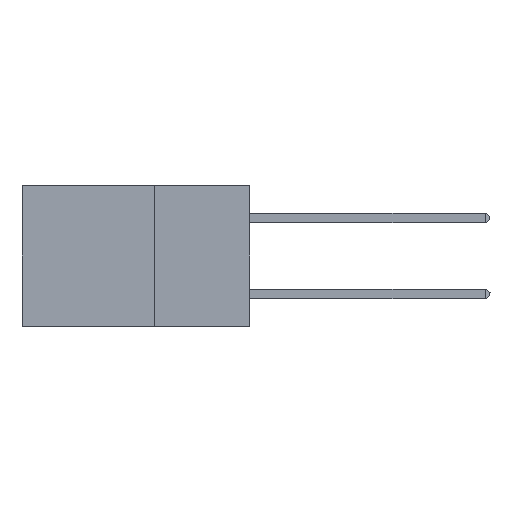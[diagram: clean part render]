
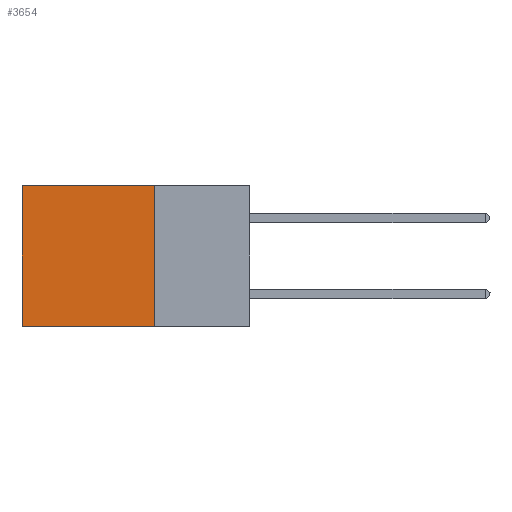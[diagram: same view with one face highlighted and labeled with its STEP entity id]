
A CAD part, left-side view. The second image highlights one B-rep face of the part: STEP entity #3654.
In plain terms, the highlighted planar face has unit normal (-1, 0, 0).
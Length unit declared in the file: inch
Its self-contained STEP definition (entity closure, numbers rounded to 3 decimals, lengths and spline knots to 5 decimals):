
#34 = LINE ( 'NONE', #11631, #18274 ) ;
#37 = PLANE ( 'NONE',  #7152 ) ;
#3406 = CARTESIAN_POINT ( 'NONE',  ( 0.2875, 0.25, 0. ) ) ;
#3477 = DIRECTION ( 'NONE',  ( 1., 0., 0. ) ) ;
#3566 = CARTESIAN_POINT ( 'NONE',  ( 0.2875, 0.25, 0. ) ) ;
#3654 = ADVANCED_FACE ( 'NONE', ( #11152 ), #37, .F. ) ;
#4020 = CARTESIAN_POINT ( 'NONE',  ( 0.2875, 0.6, 0. ) ) ;
#5907 = DIRECTION ( 'NONE',  ( 0., 1., 0. ) ) ;
#6200 = VERTEX_POINT ( 'NONE', #18949 ) ;
#6366 = VERTEX_POINT ( 'NONE', #14216 ) ;
#6969 = EDGE_CURVE ( 'NONE', #6200, #6366, #34, .T. ) ;
#7152 = AXIS2_PLACEMENT_3D ( 'NONE', #3566, #3477, #12568 ) ;
#7919 = ORIENTED_EDGE ( 'NONE', *, *, #6969, .T. ) ;
#9096 = EDGE_CURVE ( 'NONE', #6200, #17278, #19017, .T. ) ;
#9448 = ORIENTED_EDGE ( 'NONE', *, *, #17090, .T. ) ;
#9589 = DIRECTION ( 'NONE',  ( 0., 0., -1. ) ) ;
#9813 = LINE ( 'NONE', #22398, #17381 ) ;
#11152 = FACE_OUTER_BOUND ( 'NONE', #14545, .T. ) ;
#11631 = CARTESIAN_POINT ( 'NONE',  ( 0.2875, 0.25, 0. ) ) ;
#12011 = EDGE_CURVE ( 'NONE', #17278, #15014, #9813, .T. ) ;
#12568 = DIRECTION ( 'NONE',  ( 0., 0., -1. ) ) ;
#13454 = DIRECTION ( 'NONE',  ( 0., 1., 0. ) ) ;
#13642 = VECTOR ( 'NONE', #9589, 39.37008 ) ;
#14216 = CARTESIAN_POINT ( 'NONE',  ( 0.2875, 0.6, 0. ) ) ;
#14481 = LINE ( 'NONE', #4020, #13642 ) ;
#14545 = EDGE_LOOP ( 'NONE', ( #9448, #15467, #14942, #7919 ) ) ;
#14942 = ORIENTED_EDGE ( 'NONE', *, *, #9096, .F. ) ;
#15014 = VERTEX_POINT ( 'NONE', #22683 ) ;
#15467 = ORIENTED_EDGE ( 'NONE', *, *, #12011, .F. ) ;
#16002 = CARTESIAN_POINT ( 'NONE',  ( 0.2875, 0.25, -0.37 ) ) ;
#17090 = EDGE_CURVE ( 'NONE', #6366, #15014, #14481, .T. ) ;
#17278 = VERTEX_POINT ( 'NONE', #16002 ) ;
#17381 = VECTOR ( 'NONE', #5907, 39.37008 ) ;
#18274 = VECTOR ( 'NONE', #13454, 39.37008 ) ;
#18949 = CARTESIAN_POINT ( 'NONE',  ( 0.2875, 0.25, 0. ) ) ;
#19017 = LINE ( 'NONE', #3406, #19287 ) ;
#19287 = VECTOR ( 'NONE', #21292, 39.37008 ) ;
#21292 = DIRECTION ( 'NONE',  ( 0., 0., -1. ) ) ;
#22398 = CARTESIAN_POINT ( 'NONE',  ( 0.2875, 0.25, -0.37 ) ) ;
#22683 = CARTESIAN_POINT ( 'NONE',  ( 0.2875, 0.6, -0.37 ) ) ;
